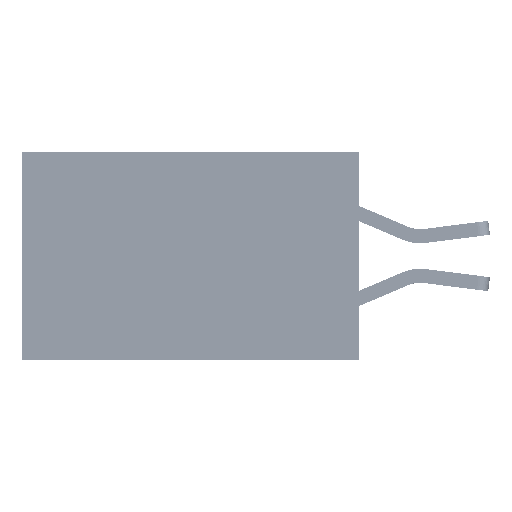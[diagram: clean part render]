
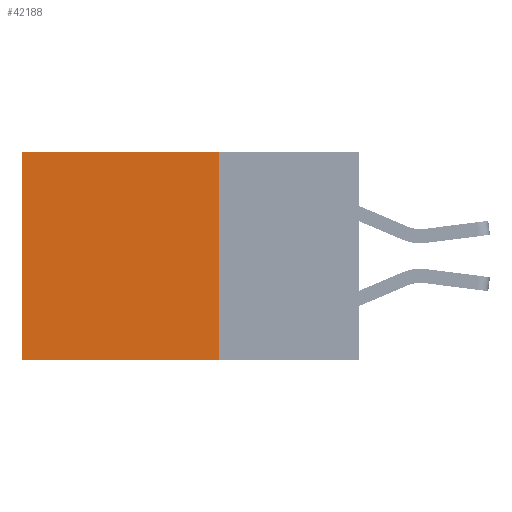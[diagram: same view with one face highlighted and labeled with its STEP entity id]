
A CAD part, left-side view. The second image highlights one B-rep face of the part: STEP entity #42188.
In plain terms, the highlighted planar face has unit normal (-1, 0, 0).
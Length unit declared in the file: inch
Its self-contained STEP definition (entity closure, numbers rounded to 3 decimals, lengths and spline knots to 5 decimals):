
#253 = VERTEX_POINT ( 'NONE', #32580 ) ;
#1893 = ORIENTED_EDGE ( 'NONE', *, *, #38556, .F. ) ;
#2003 = DIRECTION ( 'NONE',  ( 0., 1., 0. ) ) ;
#4061 = FACE_OUTER_BOUND ( 'NONE', #31791, .T. ) ;
#5469 = LINE ( 'NONE', #26956, #20492 ) ;
#5640 = DIRECTION ( 'NONE',  ( 0., 0., -1. ) ) ;
#6567 = LINE ( 'NONE', #23267, #23206 ) ;
#6615 = CARTESIAN_POINT ( 'NONE',  ( 0.2875, 0.6, -0.37 ) ) ;
#9042 = DIRECTION ( 'NONE',  ( 0., 0., -1. ) ) ;
#11682 = EDGE_CURVE ( 'NONE', #18810, #14522, #6567, .T. ) ;
#12695 = DIRECTION ( 'NONE',  ( 0., 1., 0. ) ) ;
#14522 = VERTEX_POINT ( 'NONE', #6615 ) ;
#14674 = ORIENTED_EDGE ( 'NONE', *, *, #11682, .T. ) ;
#16363 = EDGE_CURVE ( 'NONE', #41636, #14522, #29502, .T. ) ;
#17265 = CARTESIAN_POINT ( 'NONE',  ( 0.2875, 0.6, 0. ) ) ;
#17836 = VECTOR ( 'NONE', #9042, 39.37008 ) ;
#18810 = VERTEX_POINT ( 'NONE', #17265 ) ;
#20492 = VECTOR ( 'NONE', #2003, 39.37008 ) ;
#21231 = VECTOR ( 'NONE', #12695, 39.37008 ) ;
#21489 = EDGE_CURVE ( 'NONE', #253, #18810, #5469, .T. ) ;
#21793 = ORIENTED_EDGE ( 'NONE', *, *, #16363, .F. ) ;
#23206 = VECTOR ( 'NONE', #33519, 39.37008 ) ;
#23267 = CARTESIAN_POINT ( 'NONE',  ( 0.2875, 0.6, 0. ) ) ;
#26259 = CARTESIAN_POINT ( 'NONE',  ( 0.2875, 0.25, -0.37 ) ) ;
#26956 = CARTESIAN_POINT ( 'NONE',  ( 0.2875, 0.25, 0. ) ) ;
#28853 = DIRECTION ( 'NONE',  ( 1., 0., 0. ) ) ;
#29502 = LINE ( 'NONE', #42127, #21231 ) ;
#31791 = EDGE_LOOP ( 'NONE', ( #14674, #21793, #1893, #34168 ) ) ;
#32580 = CARTESIAN_POINT ( 'NONE',  ( 0.2875, 0.25, 0. ) ) ;
#33519 = DIRECTION ( 'NONE',  ( 0., 0., -1. ) ) ;
#33960 = LINE ( 'NONE', #41858, #17836 ) ;
#34168 = ORIENTED_EDGE ( 'NONE', *, *, #21489, .T. ) ;
#35192 = PLANE ( 'NONE',  #36211 ) ;
#36211 = AXIS2_PLACEMENT_3D ( 'NONE', #38721, #28853, #5640 ) ;
#38556 = EDGE_CURVE ( 'NONE', #253, #41636, #33960, .T. ) ;
#38721 = CARTESIAN_POINT ( 'NONE',  ( 0.2875, 0.25, 0. ) ) ;
#41636 = VERTEX_POINT ( 'NONE', #26259 ) ;
#41858 = CARTESIAN_POINT ( 'NONE',  ( 0.2875, 0.25, 0. ) ) ;
#42127 = CARTESIAN_POINT ( 'NONE',  ( 0.2875, 0.25, -0.37 ) ) ;
#42188 = ADVANCED_FACE ( 'NONE', ( #4061 ), #35192, .F. ) ;
